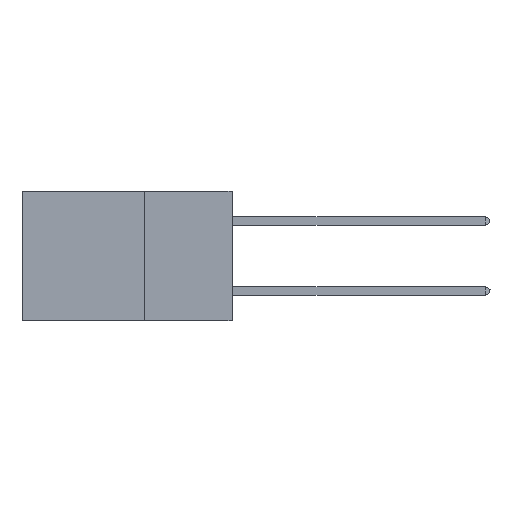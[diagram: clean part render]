
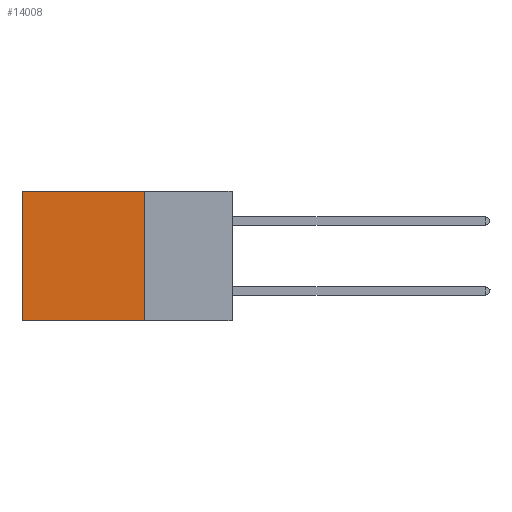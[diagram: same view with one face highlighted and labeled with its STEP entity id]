
A CAD part, left-side view. The second image highlights one B-rep face of the part: STEP entity #14008.
In plain terms, the highlighted planar face has unit normal (-1, 0, 0).
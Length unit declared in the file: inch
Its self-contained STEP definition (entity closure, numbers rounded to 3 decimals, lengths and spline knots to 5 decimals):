
#1294 = ORIENTED_EDGE ( 'NONE', *, *, #18015, .T. ) ;
#1470 = VERTEX_POINT ( 'NONE', #5496 ) ;
#1693 = VECTOR ( 'NONE', #11377, 39.37008 ) ;
#2181 = CARTESIAN_POINT ( 'NONE',  ( 0.2875, 0.25, 0. ) ) ;
#5312 = ORIENTED_EDGE ( 'NONE', *, *, #5611, .T. ) ;
#5496 = CARTESIAN_POINT ( 'NONE',  ( 0.2875, 0.6, -0.37 ) ) ;
#5611 = EDGE_CURVE ( 'NONE', #22400, #10026, #21981, .T. ) ;
#5853 = CARTESIAN_POINT ( 'NONE',  ( 0.2875, 0.25, -0.37 ) ) ;
#6025 = FACE_OUTER_BOUND ( 'NONE', #13787, .T. ) ;
#6490 = LINE ( 'NONE', #5853, #1693 ) ;
#7064 = DIRECTION ( 'NONE',  ( 1., 0., 0. ) ) ;
#7519 = EDGE_CURVE ( 'NONE', #13890, #1470, #6490, .T. ) ;
#8859 = DIRECTION ( 'NONE',  ( 0., 0., -1. ) ) ;
#8899 = CARTESIAN_POINT ( 'NONE',  ( 0.2875, 0.25, 0. ) ) ;
#9264 = ORIENTED_EDGE ( 'NONE', *, *, #16219, .F. ) ;
#9562 = CARTESIAN_POINT ( 'NONE',  ( 0.2875, 0.6, 0. ) ) ;
#10026 = VERTEX_POINT ( 'NONE', #15619 ) ;
#10988 = VECTOR ( 'NONE', #11131, 39.37008 ) ;
#11060 = CARTESIAN_POINT ( 'NONE',  ( 0.2875, 0.25, 0. ) ) ;
#11131 = DIRECTION ( 'NONE',  ( 0., 0., -1. ) ) ;
#11377 = DIRECTION ( 'NONE',  ( 0., 1., 0. ) ) ;
#12354 = CARTESIAN_POINT ( 'NONE',  ( 0.2875, 0.25, 0. ) ) ;
#13174 = CARTESIAN_POINT ( 'NONE',  ( 0.2875, 0.25, -0.37 ) ) ;
#13375 = ORIENTED_EDGE ( 'NONE', *, *, #7519, .F. ) ;
#13787 = EDGE_LOOP ( 'NONE', ( #1294, #13375, #9264, #5312 ) ) ;
#13890 = VERTEX_POINT ( 'NONE', #13174 ) ;
#14008 = ADVANCED_FACE ( 'NONE', ( #6025 ), #21324, .F. ) ;
#14752 = VECTOR ( 'NONE', #22085, 39.37008 ) ;
#15568 = LINE ( 'NONE', #9562, #14752 ) ;
#15619 = CARTESIAN_POINT ( 'NONE',  ( 0.2875, 0.6, 0. ) ) ;
#16219 = EDGE_CURVE ( 'NONE', #22400, #13890, #20511, .T. ) ;
#17233 = VECTOR ( 'NONE', #19113, 39.37008 ) ;
#18015 = EDGE_CURVE ( 'NONE', #10026, #1470, #15568, .T. ) ;
#19113 = DIRECTION ( 'NONE',  ( 0., 1., 0. ) ) ;
#20511 = LINE ( 'NONE', #11060, #10988 ) ;
#21082 = AXIS2_PLACEMENT_3D ( 'NONE', #12354, #7064, #8859 ) ;
#21324 = PLANE ( 'NONE',  #21082 ) ;
#21981 = LINE ( 'NONE', #8899, #17233 ) ;
#22085 = DIRECTION ( 'NONE',  ( 0., 0., -1. ) ) ;
#22400 = VERTEX_POINT ( 'NONE', #2181 ) ;
